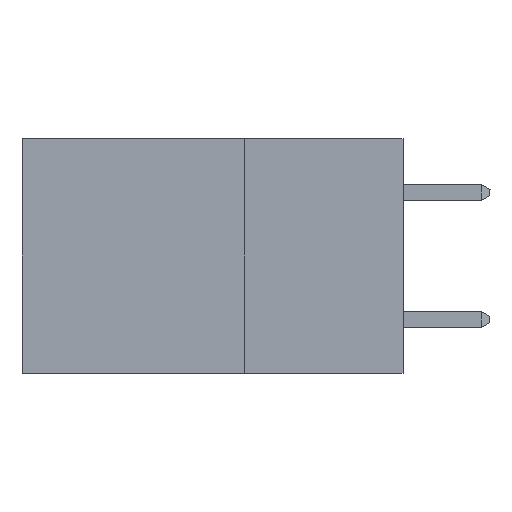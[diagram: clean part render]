
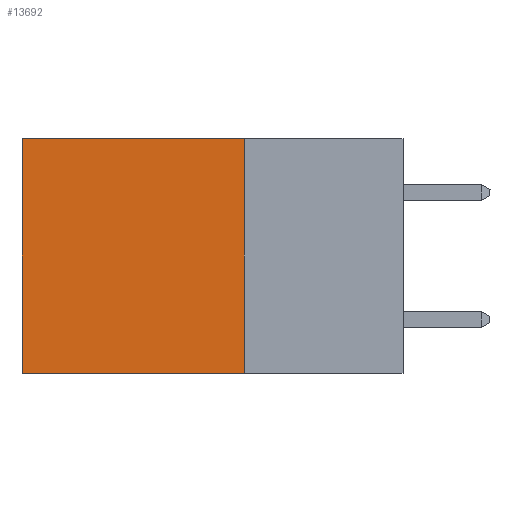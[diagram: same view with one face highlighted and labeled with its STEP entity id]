
A CAD part, left-side view. The second image highlights one B-rep face of the part: STEP entity #13692.
In plain terms, the highlighted planar face has unit normal (-1, 0, 0).
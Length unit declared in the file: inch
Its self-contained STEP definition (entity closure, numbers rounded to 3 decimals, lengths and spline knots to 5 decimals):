
#406 = DIRECTION ( 'NONE',  ( 0., 1., 0. ) ) ;
#768 = VERTEX_POINT ( 'NONE', #13162 ) ;
#2085 = CARTESIAN_POINT ( 'NONE',  ( 0.2875, 0.25, -0.37 ) ) ;
#2193 = DIRECTION ( 'NONE',  ( 0., 1., 0. ) ) ;
#2476 = CARTESIAN_POINT ( 'NONE',  ( 0.2875, 0.6, -0.37 ) ) ;
#3765 = LINE ( 'NONE', #10389, #17099 ) ;
#4095 = ORIENTED_EDGE ( 'NONE', *, *, #4529, .F. ) ;
#4529 = EDGE_CURVE ( 'NONE', #21822, #19634, #18402, .T. ) ;
#4805 = VECTOR ( 'NONE', #16583, 39.37008 ) ;
#5064 = VECTOR ( 'NONE', #2193, 39.37008 ) ;
#5598 = CARTESIAN_POINT ( 'NONE',  ( 0.2875, 0.25, 0. ) ) ;
#5843 = CARTESIAN_POINT ( 'NONE',  ( 0.2875, 0.25, 0. ) ) ;
#6196 = VECTOR ( 'NONE', #406, 39.37008 ) ;
#7276 = PLANE ( 'NONE',  #20913 ) ;
#8961 = CARTESIAN_POINT ( 'NONE',  ( 0.2875, 0.25, 0. ) ) ;
#9100 = DIRECTION ( 'NONE',  ( 0., 0., -1. ) ) ;
#9137 = CARTESIAN_POINT ( 'NONE',  ( 0.2875, 0.25, -0.37 ) ) ;
#9268 = DIRECTION ( 'NONE',  ( 1., 0., 0. ) ) ;
#9883 = VERTEX_POINT ( 'NONE', #10034 ) ;
#10034 = CARTESIAN_POINT ( 'NONE',  ( 0.2875, 0.6, 0. ) ) ;
#10389 = CARTESIAN_POINT ( 'NONE',  ( 0.2875, 0.6, 0. ) ) ;
#10812 = LINE ( 'NONE', #8961, #4805 ) ;
#12994 = EDGE_CURVE ( 'NONE', #9883, #19634, #3765, .T. ) ;
#13162 = CARTESIAN_POINT ( 'NONE',  ( 0.2875, 0.25, 0. ) ) ;
#13692 = ADVANCED_FACE ( 'NONE', ( #21697 ), #7276, .F. ) ;
#13889 = DIRECTION ( 'NONE',  ( 0., 0., -1. ) ) ;
#15334 = EDGE_CURVE ( 'NONE', #768, #21822, #10812, .T. ) ;
#15461 = ORIENTED_EDGE ( 'NONE', *, *, #15334, .F. ) ;
#15633 = ORIENTED_EDGE ( 'NONE', *, *, #12994, .T. ) ;
#16583 = DIRECTION ( 'NONE',  ( 0., 0., -1. ) ) ;
#17099 = VECTOR ( 'NONE', #13889, 39.37008 ) ;
#18402 = LINE ( 'NONE', #9137, #5064 ) ;
#19375 = EDGE_CURVE ( 'NONE', #768, #9883, #19440, .T. ) ;
#19440 = LINE ( 'NONE', #5598, #6196 ) ;
#19634 = VERTEX_POINT ( 'NONE', #2476 ) ;
#20134 = EDGE_LOOP ( 'NONE', ( #15633, #4095, #15461, #21636 ) ) ;
#20913 = AXIS2_PLACEMENT_3D ( 'NONE', #5843, #9268, #9100 ) ;
#21636 = ORIENTED_EDGE ( 'NONE', *, *, #19375, .T. ) ;
#21697 = FACE_OUTER_BOUND ( 'NONE', #20134, .T. ) ;
#21822 = VERTEX_POINT ( 'NONE', #2085 ) ;
